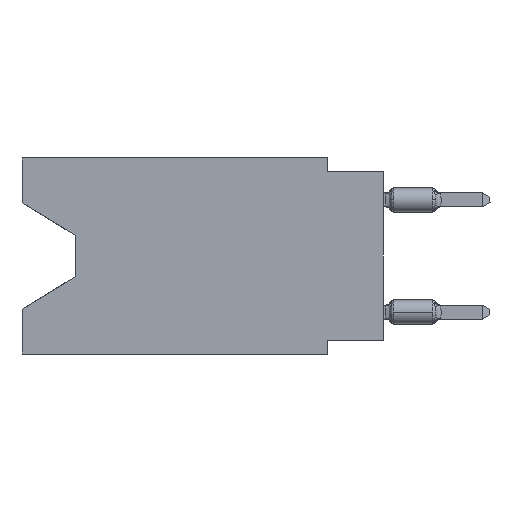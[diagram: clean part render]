
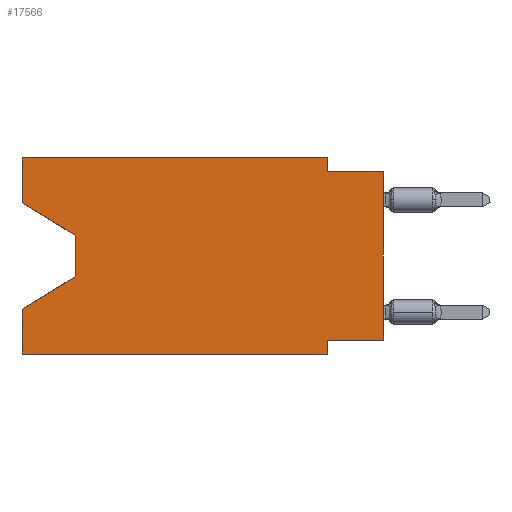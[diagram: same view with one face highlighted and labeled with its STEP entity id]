
A CAD part, left-side view. The second image highlights one B-rep face of the part: STEP entity #17566.
In plain terms, the highlighted planar face has unit normal (-1, 0, 0).
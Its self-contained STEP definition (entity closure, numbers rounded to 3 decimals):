
#101 = DIRECTION ( 'NONE',  ( 0., 0., 1. ) ) ;
#2378 = CARTESIAN_POINT ( 'NONE',  ( 0., 16.383, 0. ) ) ;
#3461 = ORIENTED_EDGE ( 'NONE', *, *, #34422, .F. ) ;
#3567 = VECTOR ( 'NONE', #6020, 1000. ) ;
#4142 = AXIS2_PLACEMENT_3D ( 'NONE', #36764, #6589, #27652 ) ;
#5120 = CARTESIAN_POINT ( 'NONE',  ( 0., 2.54, -8.89 ) ) ;
#5121 = LINE ( 'NONE', #20227, #5586 ) ;
#5586 = VECTOR ( 'NONE', #38464, 1000. ) ;
#6020 = DIRECTION ( 'NONE',  ( 0., 0., -1. ) ) ;
#6265 = VERTEX_POINT ( 'NONE', #30282 ) ;
#6589 = DIRECTION ( 'NONE',  ( 1., 0., 0. ) ) ;
#6640 = EDGE_CURVE ( 'NONE', #6265, #20383, #18404, .T. ) ;
#7686 = ORIENTED_EDGE ( 'NONE', *, *, #30741, .F. ) ;
#8720 = VECTOR ( 'NONE', #19981, 1000. ) ;
#8990 = VECTOR ( 'NONE', #30070, 1000. ) ;
#9842 = LINE ( 'NONE', #18974, #15017 ) ;
#10218 = ORIENTED_EDGE ( 'NONE', *, *, #10350, .F. ) ;
#10350 = EDGE_CURVE ( 'NONE', #30414, #26189, #5121, .T. ) ;
#10422 = LINE ( 'NONE', #22715, #27890 ) ;
#11227 = VERTEX_POINT ( 'NONE', #33577 ) ;
#11464 = VECTOR ( 'NONE', #101, 1000. ) ;
#11868 = CARTESIAN_POINT ( 'NONE',  ( 0., 2.54, -0.635 ) ) ;
#11984 = VERTEX_POINT ( 'NONE', #5120 ) ;
#12243 = CARTESIAN_POINT ( 'NONE',  ( 0., 16.383, 0. ) ) ;
#12702 = ORIENTED_EDGE ( 'NONE', *, *, #6640, .T. ) ;
#12708 = EDGE_CURVE ( 'NONE', #30974, #6265, #15519, .T. ) ;
#12961 = FACE_OUTER_BOUND ( 'NONE', #28399, .T. ) ;
#13215 = DIRECTION ( 'NONE',  ( 0., -0.855, -0.519 ) ) ;
#13464 = LINE ( 'NONE', #12243, #11464 ) ;
#13681 = VECTOR ( 'NONE', #31663, 1000. ) ;
#14174 = VERTEX_POINT ( 'NONE', #35227 ) ;
#14994 = CARTESIAN_POINT ( 'NONE',  ( 0., 0., -8.255 ) ) ;
#15017 = VECTOR ( 'NONE', #21936, 1000. ) ;
#15519 = LINE ( 'NONE', #26821, #25815 ) ;
#16475 = CARTESIAN_POINT ( 'NONE',  ( 0., 2.54, 0. ) ) ;
#16983 = LINE ( 'NONE', #26281, #13681 ) ;
#17196 = CARTESIAN_POINT ( 'NONE',  ( 0., 0., 0. ) ) ;
#17282 = EDGE_CURVE ( 'NONE', #11227, #11984, #16983, .T. ) ;
#17566 = ADVANCED_FACE ( 'NONE', ( #12961 ), #21872, .F. ) ;
#17863 = VERTEX_POINT ( 'NONE', #29990 ) ;
#18331 = CARTESIAN_POINT ( 'NONE',  ( 0., 16.383, -2.038 ) ) ;
#18404 = LINE ( 'NONE', #27512, #21557 ) ;
#18519 = ORIENTED_EDGE ( 'NONE', *, *, #37679, .T. ) ;
#18682 = ORIENTED_EDGE ( 'NONE', *, *, #17282, .F. ) ;
#18974 = CARTESIAN_POINT ( 'NONE',  ( 0., 16.383, 0. ) ) ;
#19981 = DIRECTION ( 'NONE',  ( 0., -1., 0. ) ) ;
#19983 = ORIENTED_EDGE ( 'NONE', *, *, #12708, .T. ) ;
#20227 = CARTESIAN_POINT ( 'NONE',  ( 0., 0., -0.635 ) ) ;
#20383 = VERTEX_POINT ( 'NONE', #33936 ) ;
#20426 = LINE ( 'NONE', #2378, #24893 ) ;
#20601 = VERTEX_POINT ( 'NONE', #16475 ) ;
#21557 = VECTOR ( 'NONE', #24147, 1000. ) ;
#21872 = PLANE ( 'NONE',  #4142 ) ;
#21884 = ORIENTED_EDGE ( 'NONE', *, *, #39240, .T. ) ;
#21936 = DIRECTION ( 'NONE',  ( 0., -1., 0. ) ) ;
#21978 = VERTEX_POINT ( 'NONE', #18331 ) ;
#22715 = CARTESIAN_POINT ( 'NONE',  ( 0., 16.383, -2.038 ) ) ;
#24147 = DIRECTION ( 'NONE',  ( 0., 0.855, -0.519 ) ) ;
#24893 = VECTOR ( 'NONE', #26583, 1000. ) ;
#24943 = EDGE_CURVE ( 'NONE', #17863, #11227, #29873, .T. ) ;
#25293 = ORIENTED_EDGE ( 'NONE', *, *, #30562, .F. ) ;
#25815 = VECTOR ( 'NONE', #27023, 1000. ) ;
#25935 = EDGE_CURVE ( 'NONE', #17863, #26189, #35044, .T. ) ;
#26189 = VERTEX_POINT ( 'NONE', #33462 ) ;
#26281 = CARTESIAN_POINT ( 'NONE',  ( 0., 2.54, -8.89 ) ) ;
#26583 = DIRECTION ( 'NONE',  ( 0., 0., 1. ) ) ;
#26821 = CARTESIAN_POINT ( 'NONE',  ( 0., 13.97, -3.505 ) ) ;
#26887 = ORIENTED_EDGE ( 'NONE', *, *, #24943, .F. ) ;
#26892 = VERTEX_POINT ( 'NONE', #39113 ) ;
#27023 = DIRECTION ( 'NONE',  ( 0., 0., -1. ) ) ;
#27425 = VECTOR ( 'NONE', #29299, 1000. ) ;
#27457 = CARTESIAN_POINT ( 'NONE',  ( 0., 2.54, 0. ) ) ;
#27512 = CARTESIAN_POINT ( 'NONE',  ( 0., 13.97, -5.385 ) ) ;
#27652 = DIRECTION ( 'NONE',  ( 0., 0., -1. ) ) ;
#27890 = VECTOR ( 'NONE', #13215, 1000. ) ;
#28399 = EDGE_LOOP ( 'NONE', ( #21884, #19983, #12702, #37178, #18519, #18682, #26887, #33404, #10218, #7686, #25293, #3461 ) ) ;
#28874 = EDGE_CURVE ( 'NONE', #14174, #20383, #13464, .T. ) ;
#29299 = DIRECTION ( 'NONE',  ( 0., 0., 1. ) ) ;
#29873 = LINE ( 'NONE', #14994, #8990 ) ;
#29990 = CARTESIAN_POINT ( 'NONE',  ( 0., 0., -8.255 ) ) ;
#30070 = DIRECTION ( 'NONE',  ( 0., 1., 0. ) ) ;
#30282 = CARTESIAN_POINT ( 'NONE',  ( 0., 13.97, -5.385 ) ) ;
#30414 = VERTEX_POINT ( 'NONE', #11868 ) ;
#30562 = EDGE_CURVE ( 'NONE', #26892, #20601, #9842, .T. ) ;
#30741 = EDGE_CURVE ( 'NONE', #20601, #30414, #36388, .T. ) ;
#30974 = VERTEX_POINT ( 'NONE', #31168 ) ;
#31168 = CARTESIAN_POINT ( 'NONE',  ( 0., 13.97, -3.505 ) ) ;
#31663 = DIRECTION ( 'NONE',  ( 0., 0., -1. ) ) ;
#33404 = ORIENTED_EDGE ( 'NONE', *, *, #25935, .T. ) ;
#33462 = CARTESIAN_POINT ( 'NONE',  ( 0., 0., -0.635 ) ) ;
#33577 = CARTESIAN_POINT ( 'NONE',  ( 0., 2.54, -8.255 ) ) ;
#33936 = CARTESIAN_POINT ( 'NONE',  ( 0., 16.383, -6.852 ) ) ;
#34422 = EDGE_CURVE ( 'NONE', #21978, #26892, #20426, .T. ) ;
#35044 = LINE ( 'NONE', #17196, #27425 ) ;
#35046 = LINE ( 'NONE', #38016, #8720 ) ;
#35227 = CARTESIAN_POINT ( 'NONE',  ( 0., 16.383, -8.89 ) ) ;
#36388 = LINE ( 'NONE', #27457, #3567 ) ;
#36764 = CARTESIAN_POINT ( 'NONE',  ( 0., 16.383, 0. ) ) ;
#37178 = ORIENTED_EDGE ( 'NONE', *, *, #28874, .F. ) ;
#37679 = EDGE_CURVE ( 'NONE', #14174, #11984, #35046, .T. ) ;
#38016 = CARTESIAN_POINT ( 'NONE',  ( 0., 16.383, -8.89 ) ) ;
#38464 = DIRECTION ( 'NONE',  ( 0., -1., 0. ) ) ;
#39113 = CARTESIAN_POINT ( 'NONE',  ( 0., 16.383, 0. ) ) ;
#39240 = EDGE_CURVE ( 'NONE', #21978, #30974, #10422, .T. ) ;
